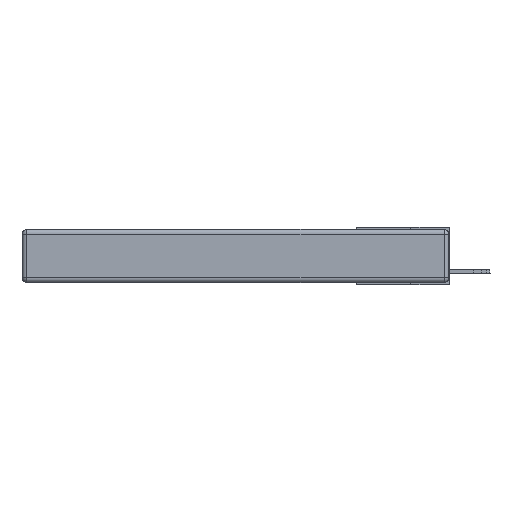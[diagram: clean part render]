
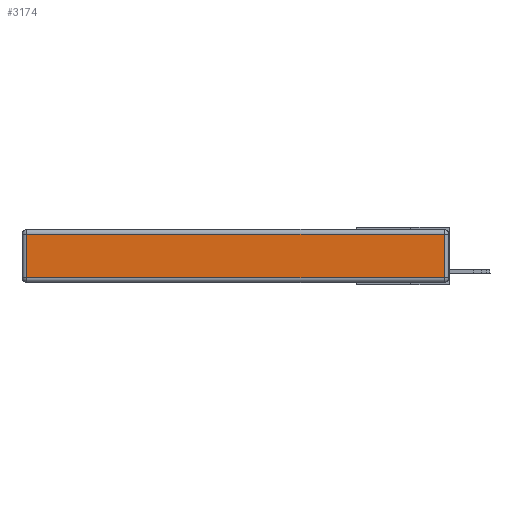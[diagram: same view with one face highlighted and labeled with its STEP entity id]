
A CAD part, left-side view. The second image highlights one B-rep face of the part: STEP entity #3174.
In plain terms, the highlighted planar face has unit normal (-1, 0, 0).
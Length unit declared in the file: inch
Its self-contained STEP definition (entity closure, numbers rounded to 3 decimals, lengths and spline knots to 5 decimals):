
#224 = VERTEX_POINT ( 'NONE', #17472 ) ;
#231 = ORIENTED_EDGE ( 'NONE', *, *, #18621, .T. ) ;
#314 = CARTESIAN_POINT ( 'NONE',  ( 0., 2.75, -0.03 ) ) ;
#411 = VECTOR ( 'NONE', #16060, 39.37008 ) ;
#1948 = CARTESIAN_POINT ( 'NONE',  ( 0., 0.03, -0.343 ) ) ;
#2614 = ORIENTED_EDGE ( 'NONE', *, *, #3008, .T. ) ;
#2840 = CARTESIAN_POINT ( 'NONE',  ( 0., 0., -0.343 ) ) ;
#2880 = ORIENTED_EDGE ( 'NONE', *, *, #18624, .T. ) ;
#3008 = EDGE_CURVE ( 'NONE', #224, #16662, #13047, .T. ) ;
#3174 = ADVANCED_FACE ( 'NONE', ( #12742 ), #19780, .T. ) ;
#4990 = CARTESIAN_POINT ( 'NONE',  ( 0., 0.03, -0.03 ) ) ;
#5035 = ORIENTED_EDGE ( 'NONE', *, *, #13294, .T. ) ;
#5074 = VECTOR ( 'NONE', #19187, 39.37008 ) ;
#6579 = DIRECTION ( 'NONE',  ( 0., 0., 1. ) ) ;
#7963 = EDGE_LOOP ( 'NONE', ( #2614, #231, #2880, #5035 ) ) ;
#8005 = DIRECTION ( 'NONE',  ( 0., -1., 0. ) ) ;
#9796 = CARTESIAN_POINT ( 'NONE',  ( 0., 0.03, -0.313 ) ) ;
#12742 = FACE_OUTER_BOUND ( 'NONE', #7963, .T. ) ;
#13047 = LINE ( 'NONE', #17052, #23825 ) ;
#13294 = EDGE_CURVE ( 'NONE', #13730, #224, #19923, .T. ) ;
#13730 = VERTEX_POINT ( 'NONE', #19896 ) ;
#14044 = VERTEX_POINT ( 'NONE', #4990 ) ;
#14168 = CARTESIAN_POINT ( 'NONE',  ( 0., 2.72, -0.343 ) ) ;
#15866 = DIRECTION ( 'NONE',  ( -1., 0., 0. ) ) ;
#16060 = DIRECTION ( 'NONE',  ( 0., 0., -1. ) ) ;
#16662 = VERTEX_POINT ( 'NONE', #9796 ) ;
#17052 = CARTESIAN_POINT ( 'NONE',  ( 0., 0., -0.313 ) ) ;
#17472 = CARTESIAN_POINT ( 'NONE',  ( 0., 2.72, -0.313 ) ) ;
#17609 = LINE ( 'NONE', #1948, #17880 ) ;
#17880 = VECTOR ( 'NONE', #22970, 39.37008 ) ;
#18370 = AXIS2_PLACEMENT_3D ( 'NONE', #2840, #15866, #6579 ) ;
#18621 = EDGE_CURVE ( 'NONE', #16662, #14044, #17609, .T. ) ;
#18624 = EDGE_CURVE ( 'NONE', #14044, #13730, #19951, .T. ) ;
#19187 = DIRECTION ( 'NONE',  ( 0., 1., 0. ) ) ;
#19780 = PLANE ( 'NONE',  #18370 ) ;
#19896 = CARTESIAN_POINT ( 'NONE',  ( 0., 2.72, -0.03 ) ) ;
#19923 = LINE ( 'NONE', #14168, #411 ) ;
#19951 = LINE ( 'NONE', #314, #5074 ) ;
#22970 = DIRECTION ( 'NONE',  ( 0., 0., 1. ) ) ;
#23825 = VECTOR ( 'NONE', #8005, 39.37008 ) ;
